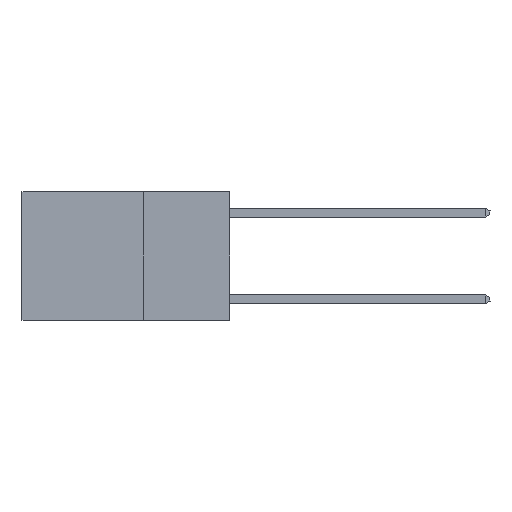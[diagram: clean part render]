
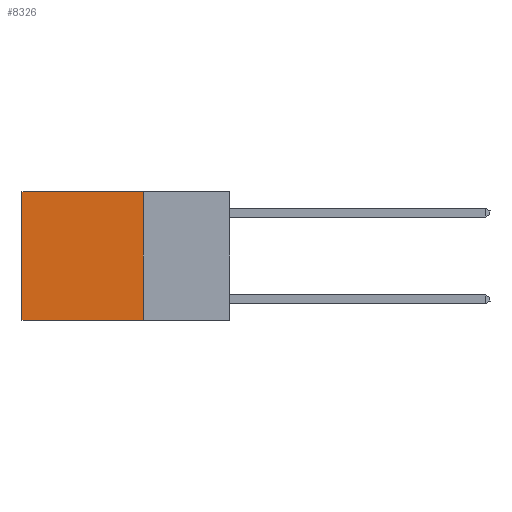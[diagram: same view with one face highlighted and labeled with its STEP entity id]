
A CAD part, left-side view. The second image highlights one B-rep face of the part: STEP entity #8326.
In plain terms, the highlighted planar face has unit normal (-1, 0, 0).
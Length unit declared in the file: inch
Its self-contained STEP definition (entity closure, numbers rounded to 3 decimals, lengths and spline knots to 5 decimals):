
#148 = ORIENTED_EDGE ( 'NONE', *, *, #4208, .T. ) ;
#452 = DIRECTION ( 'NONE',  ( 0., 0., -1. ) ) ;
#500 = DIRECTION ( 'NONE',  ( 0., 0., -1. ) ) ;
#786 = VECTOR ( 'NONE', #452, 39.37008 ) ;
#796 = DIRECTION ( 'NONE',  ( 0., 0., -1. ) ) ;
#1252 = LINE ( 'NONE', #9937, #786 ) ;
#1537 = FACE_OUTER_BOUND ( 'NONE', #7012, .T. ) ;
#1674 = EDGE_CURVE ( 'NONE', #7858, #4278, #1252, .T. ) ;
#2580 = CARTESIAN_POINT ( 'NONE',  ( 0.2625, 0.25, -0.37 ) ) ;
#2957 = EDGE_CURVE ( 'NONE', #4278, #4084, #6391, .T. ) ;
#3185 = VECTOR ( 'NONE', #500, 39.37008 ) ;
#3452 = DIRECTION ( 'NONE',  ( 1., 0., 0. ) ) ;
#4084 = VERTEX_POINT ( 'NONE', #9947 ) ;
#4208 = EDGE_CURVE ( 'NONE', #7858, #8025, #6361, .T. ) ;
#4278 = VERTEX_POINT ( 'NONE', #9247 ) ;
#4674 = CARTESIAN_POINT ( 'NONE',  ( 0.2625, 0.25, 0. ) ) ;
#6266 = PLANE ( 'NONE',  #9630 ) ;
#6361 = LINE ( 'NONE', #4674, #9815 ) ;
#6391 = LINE ( 'NONE', #2580, #8756 ) ;
#6704 = CARTESIAN_POINT ( 'NONE',  ( 0.2625, 0.6, 0. ) ) ;
#7012 = EDGE_LOOP ( 'NONE', ( #10162, #7019, #8227, #148 ) ) ;
#7019 = ORIENTED_EDGE ( 'NONE', *, *, #2957, .F. ) ;
#7193 = CARTESIAN_POINT ( 'NONE',  ( 0.2625, 0.25, 0. ) ) ;
#7858 = VERTEX_POINT ( 'NONE', #8507 ) ;
#8025 = VERTEX_POINT ( 'NONE', #6704 ) ;
#8141 = LINE ( 'NONE', #10990, #3185 ) ;
#8227 = ORIENTED_EDGE ( 'NONE', *, *, #1674, .F. ) ;
#8326 = ADVANCED_FACE ( 'NONE', ( #1537 ), #6266, .F. ) ;
#8507 = CARTESIAN_POINT ( 'NONE',  ( 0.2625, 0.25, 0. ) ) ;
#8756 = VECTOR ( 'NONE', #9341, 39.37008 ) ;
#9247 = CARTESIAN_POINT ( 'NONE',  ( 0.2625, 0.25, -0.37 ) ) ;
#9341 = DIRECTION ( 'NONE',  ( 0., 1., 0. ) ) ;
#9630 = AXIS2_PLACEMENT_3D ( 'NONE', #7193, #3452, #796 ) ;
#9815 = VECTOR ( 'NONE', #12297, 39.37008 ) ;
#9937 = CARTESIAN_POINT ( 'NONE',  ( 0.2625, 0.25, 0. ) ) ;
#9947 = CARTESIAN_POINT ( 'NONE',  ( 0.2625, 0.6, -0.37 ) ) ;
#10162 = ORIENTED_EDGE ( 'NONE', *, *, #10849, .T. ) ;
#10849 = EDGE_CURVE ( 'NONE', #8025, #4084, #8141, .T. ) ;
#10990 = CARTESIAN_POINT ( 'NONE',  ( 0.2625, 0.6, 0. ) ) ;
#12297 = DIRECTION ( 'NONE',  ( 0., 1., 0. ) ) ;
